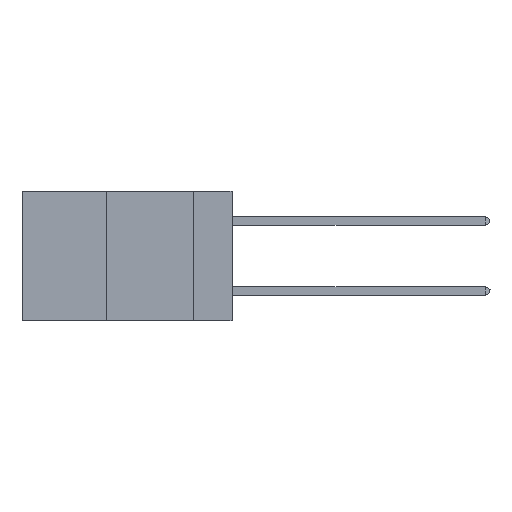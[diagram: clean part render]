
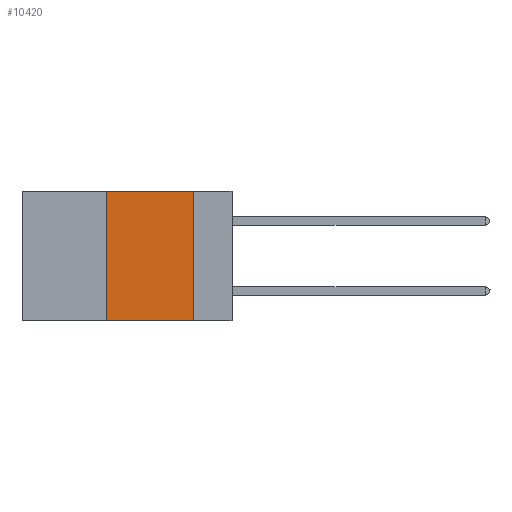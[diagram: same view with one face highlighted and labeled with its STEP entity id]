
A CAD part, left-side view. The second image highlights one B-rep face of the part: STEP entity #10420.
In plain terms, the highlighted planar face has unit normal (-1, 0, 0).
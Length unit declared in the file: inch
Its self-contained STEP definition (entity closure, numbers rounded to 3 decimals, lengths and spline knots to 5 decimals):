
#189 = CARTESIAN_POINT ( 'NONE',  ( 0., 0.36, -0.37 ) ) ;
#547 = VECTOR ( 'NONE', #29927, 39.37008 ) ;
#1442 = ORIENTED_EDGE ( 'NONE', *, *, #36021, .F. ) ;
#2943 = EDGE_LOOP ( 'NONE', ( #8925, #1442, #37083, #30298 ) ) ;
#5643 = VERTEX_POINT ( 'NONE', #14815 ) ;
#5712 = CARTESIAN_POINT ( 'NONE',  ( 0., 0.6, 0. ) ) ;
#6555 = LINE ( 'NONE', #19871, #21770 ) ;
#8925 = ORIENTED_EDGE ( 'NONE', *, *, #9316, .F. ) ;
#9316 = EDGE_CURVE ( 'NONE', #10707, #25790, #38142, .T. ) ;
#10420 = ADVANCED_FACE ( 'NONE', ( #10965 ), #18214, .F. ) ;
#10707 = VERTEX_POINT ( 'NONE', #28798 ) ;
#10965 = FACE_OUTER_BOUND ( 'NONE', #2943, .T. ) ;
#11723 = EDGE_CURVE ( 'NONE', #17230, #5643, #6555, .T. ) ;
#14815 = CARTESIAN_POINT ( 'NONE',  ( 0., 0.36, 0. ) ) ;
#15112 = CARTESIAN_POINT ( 'NONE',  ( 0., 0.11, -0.37 ) ) ;
#17230 = VERTEX_POINT ( 'NONE', #189 ) ;
#18214 = PLANE ( 'NONE',  #27795 ) ;
#19871 = CARTESIAN_POINT ( 'NONE',  ( 0., 0.36, 0. ) ) ;
#21770 = VECTOR ( 'NONE', #34808, 39.37008 ) ;
#22066 = LINE ( 'NONE', #33046, #28276 ) ;
#23745 = DIRECTION ( 'NONE',  ( 0., -1., 0. ) ) ;
#25790 = VERTEX_POINT ( 'NONE', #15112 ) ;
#27148 = CARTESIAN_POINT ( 'NONE',  ( 0., 0.11, 0. ) ) ;
#27795 = AXIS2_PLACEMENT_3D ( 'NONE', #5712, #33116, #32992 ) ;
#28276 = VECTOR ( 'NONE', #23745, 39.37008 ) ;
#28798 = CARTESIAN_POINT ( 'NONE',  ( 0., 0.11, 0. ) ) ;
#29927 = DIRECTION ( 'NONE',  ( 0., 0., -1. ) ) ;
#30298 = ORIENTED_EDGE ( 'NONE', *, *, #37092, .T. ) ;
#30729 = LINE ( 'NONE', #34606, #32634 ) ;
#31269 = DIRECTION ( 'NONE',  ( 0., -1., 0. ) ) ;
#32634 = VECTOR ( 'NONE', #31269, 39.37008 ) ;
#32992 = DIRECTION ( 'NONE',  ( 0., 0., -1. ) ) ;
#33046 = CARTESIAN_POINT ( 'NONE',  ( 0., 0.6, -0.37 ) ) ;
#33116 = DIRECTION ( 'NONE',  ( 1., 0., 0. ) ) ;
#34606 = CARTESIAN_POINT ( 'NONE',  ( 0., 0.6, 0. ) ) ;
#34808 = DIRECTION ( 'NONE',  ( 0., 0., 1. ) ) ;
#36021 = EDGE_CURVE ( 'NONE', #5643, #10707, #30729, .T. ) ;
#37083 = ORIENTED_EDGE ( 'NONE', *, *, #11723, .F. ) ;
#37092 = EDGE_CURVE ( 'NONE', #17230, #25790, #22066, .T. ) ;
#38142 = LINE ( 'NONE', #27148, #547 ) ;
